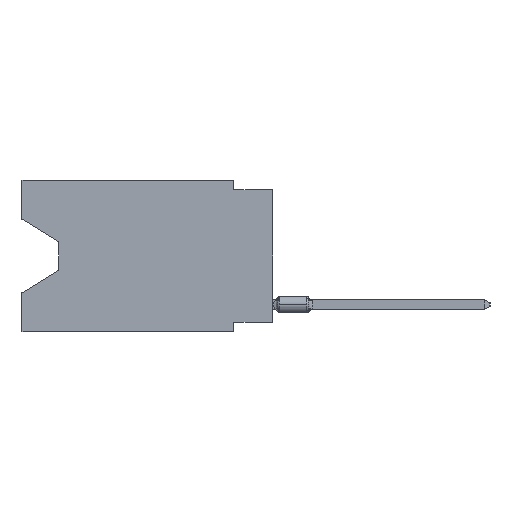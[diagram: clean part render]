
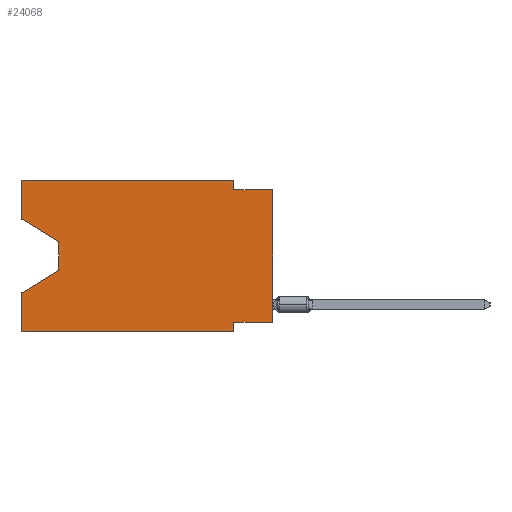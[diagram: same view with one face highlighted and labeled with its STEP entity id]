
A CAD part, left-side view. The second image highlights one B-rep face of the part: STEP entity #24068.
In plain terms, the highlighted planar face has unit normal (-1, 0, 0).
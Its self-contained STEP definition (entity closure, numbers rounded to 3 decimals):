
#17 = ORIENTED_EDGE ( 'NONE', *, *, #21297, .T. ) ;
#124 = VERTEX_POINT ( 'NONE', #58480 ) ;
#221 = VECTOR ( 'NONE', #21077, 1000. ) ;
#1026 = CARTESIAN_POINT ( 'NONE',  ( 0., 0., -0.635 ) ) ;
#1356 = LINE ( 'NONE', #67467, #20884 ) ;
#1847 = ORIENTED_EDGE ( 'NONE', *, *, #46155, .F. ) ;
#2629 = ORIENTED_EDGE ( 'NONE', *, *, #65726, .F. ) ;
#3691 = ORIENTED_EDGE ( 'NONE', *, *, #34728, .T. ) ;
#5023 = CARTESIAN_POINT ( 'NONE',  ( 0., 13.97, -5.893 ) ) ;
#10406 = CARTESIAN_POINT ( 'NONE',  ( 0., 13.97, -4.013 ) ) ;
#10746 = LINE ( 'NONE', #15737, #221 ) ;
#13681 = VERTEX_POINT ( 'NONE', #19581 ) ;
#15737 = CARTESIAN_POINT ( 'NONE',  ( 0., 16.383, -2.546 ) ) ;
#16040 = LINE ( 'NONE', #27062, #33808 ) ;
#17050 = EDGE_CURVE ( 'NONE', #27678, #64000, #19194, .T. ) ;
#17085 = CARTESIAN_POINT ( 'NONE',  ( 0., 0., -9.271 ) ) ;
#17692 = DIRECTION ( 'NONE',  ( 0., -1., 0. ) ) ;
#19194 = LINE ( 'NONE', #66882, #19429 ) ;
#19231 = DIRECTION ( 'NONE',  ( 0., 0., -1. ) ) ;
#19429 = VECTOR ( 'NONE', #57601, 1000. ) ;
#19581 = CARTESIAN_POINT ( 'NONE',  ( 0., 13.97, -4.013 ) ) ;
#20653 = DIRECTION ( 'NONE',  ( 0., 0., -1. ) ) ;
#20884 = VECTOR ( 'NONE', #17692, 1000. ) ;
#21077 = DIRECTION ( 'NONE',  ( 0., -0.855, -0.519 ) ) ;
#21142 = VECTOR ( 'NONE', #41375, 1000. ) ;
#21297 = EDGE_CURVE ( 'NONE', #68445, #124, #57919, .T. ) ;
#21388 = VERTEX_POINT ( 'NONE', #47588 ) ;
#21980 = EDGE_CURVE ( 'NONE', #68445, #21388, #50448, .T. ) ;
#21984 = VECTOR ( 'NONE', #36473, 1000. ) ;
#22849 = ORIENTED_EDGE ( 'NONE', *, *, #21980, .F. ) ;
#23095 = DIRECTION ( 'NONE',  ( 0., 0., 1. ) ) ;
#23615 = VERTEX_POINT ( 'NONE', #55124 ) ;
#23809 = EDGE_CURVE ( 'NONE', #13681, #24211, #70156, .T. ) ;
#24068 = ADVANCED_FACE ( 'NONE', ( #45902 ), #55889, .F. ) ;
#24211 = VERTEX_POINT ( 'NONE', #34907 ) ;
#25310 = DIRECTION ( 'NONE',  ( 0., 0.855, -0.519 ) ) ;
#25467 = EDGE_CURVE ( 'NONE', #29958, #57951, #69388, .T. ) ;
#25498 = VECTOR ( 'NONE', #25310, 1000. ) ;
#25687 = LINE ( 'NONE', #63403, #52208 ) ;
#27062 = CARTESIAN_POINT ( 'NONE',  ( 0., 2.54, -9.906 ) ) ;
#27487 = EDGE_LOOP ( 'NONE', ( #3691, #44027, #43756, #22849, #17, #68698, #41922, #69573, #2629, #48089, #1847, #38652 ) ) ;
#27678 = VERTEX_POINT ( 'NONE', #36654 ) ;
#27753 = VECTOR ( 'NONE', #23095, 1000. ) ;
#29958 = VERTEX_POINT ( 'NONE', #58519 ) ;
#30623 = EDGE_CURVE ( 'NONE', #63298, #23615, #44476, .T. ) ;
#32055 = LINE ( 'NONE', #5023, #25498 ) ;
#32377 = CARTESIAN_POINT ( 'NONE',  ( 0., 16.383, 0. ) ) ;
#33710 = CARTESIAN_POINT ( 'NONE',  ( 0., 16.383, -9.906 ) ) ;
#33808 = VECTOR ( 'NONE', #59084, 1000. ) ;
#34728 = EDGE_CURVE ( 'NONE', #27678, #13681, #10746, .T. ) ;
#34907 = CARTESIAN_POINT ( 'NONE',  ( 0., 13.97, -5.893 ) ) ;
#36473 = DIRECTION ( 'NONE',  ( 0., 0., 1. ) ) ;
#36654 = CARTESIAN_POINT ( 'NONE',  ( 0., 16.383, -2.546 ) ) ;
#36928 = CARTESIAN_POINT ( 'NONE',  ( 0., 16.383, -9.906 ) ) ;
#37163 = LINE ( 'NONE', #65257, #21984 ) ;
#37891 = VECTOR ( 'NONE', #68950, 1000. ) ;
#38652 = ORIENTED_EDGE ( 'NONE', *, *, #17050, .F. ) ;
#38673 = CARTESIAN_POINT ( 'NONE',  ( 0., 0., -9.271 ) ) ;
#41375 = DIRECTION ( 'NONE',  ( 0., 0., -1. ) ) ;
#41922 = ORIENTED_EDGE ( 'NONE', *, *, #30623, .F. ) ;
#43756 = ORIENTED_EDGE ( 'NONE', *, *, #66244, .T. ) ;
#44027 = ORIENTED_EDGE ( 'NONE', *, *, #23809, .T. ) ;
#44476 = LINE ( 'NONE', #17085, #60028 ) ;
#45902 = FACE_OUTER_BOUND ( 'NONE', #27487, .T. ) ;
#46155 = EDGE_CURVE ( 'NONE', #64000, #29958, #25687, .T. ) ;
#46250 = DIRECTION ( 'NONE',  ( 1., 0., 0. ) ) ;
#47370 = DIRECTION ( 'NONE',  ( 0., -1., 0. ) ) ;
#47588 = CARTESIAN_POINT ( 'NONE',  ( 0., 16.383, -7.36 ) ) ;
#47671 = CARTESIAN_POINT ( 'NONE',  ( 0., 2.54, 0. ) ) ;
#48089 = ORIENTED_EDGE ( 'NONE', *, *, #25467, .F. ) ;
#49818 = CARTESIAN_POINT ( 'NONE',  ( 0., 2.54, -0.635 ) ) ;
#50448 = LINE ( 'NONE', #55802, #27753 ) ;
#52208 = VECTOR ( 'NONE', #47370, 1000. ) ;
#53442 = EDGE_CURVE ( 'NONE', #23615, #124, #16040, .T. ) ;
#55124 = CARTESIAN_POINT ( 'NONE',  ( 0., 2.54, -9.271 ) ) ;
#55802 = CARTESIAN_POINT ( 'NONE',  ( 0., 16.383, 0. ) ) ;
#55889 = PLANE ( 'NONE',  #67745 ) ;
#57601 = DIRECTION ( 'NONE',  ( 0., 0., 1. ) ) ;
#57919 = LINE ( 'NONE', #36928, #37891 ) ;
#57951 = VERTEX_POINT ( 'NONE', #49818 ) ;
#58480 = CARTESIAN_POINT ( 'NONE',  ( 0., 2.54, -9.906 ) ) ;
#58519 = CARTESIAN_POINT ( 'NONE',  ( 0., 2.54, 0. ) ) ;
#59084 = DIRECTION ( 'NONE',  ( 0., 0., -1. ) ) ;
#60028 = VECTOR ( 'NONE', #65118, 1000. ) ;
#63006 = EDGE_CURVE ( 'NONE', #63298, #66802, #37163, .T. ) ;
#63298 = VERTEX_POINT ( 'NONE', #38673 ) ;
#63403 = CARTESIAN_POINT ( 'NONE',  ( 0., 16.383, 0. ) ) ;
#64000 = VERTEX_POINT ( 'NONE', #32377 ) ;
#64204 = VECTOR ( 'NONE', #20653, 1000. ) ;
#65118 = DIRECTION ( 'NONE',  ( 0., 1., 0. ) ) ;
#65257 = CARTESIAN_POINT ( 'NONE',  ( 0., 0., 0. ) ) ;
#65726 = EDGE_CURVE ( 'NONE', #57951, #66802, #1356, .T. ) ;
#66244 = EDGE_CURVE ( 'NONE', #24211, #21388, #32055, .T. ) ;
#66802 = VERTEX_POINT ( 'NONE', #1026 ) ;
#66882 = CARTESIAN_POINT ( 'NONE',  ( 0., 16.383, 0. ) ) ;
#67467 = CARTESIAN_POINT ( 'NONE',  ( 0., 0., -0.635 ) ) ;
#67601 = CARTESIAN_POINT ( 'NONE',  ( 0., 16.383, 0. ) ) ;
#67745 = AXIS2_PLACEMENT_3D ( 'NONE', #67601, #46250, #19231 ) ;
#68445 = VERTEX_POINT ( 'NONE', #33710 ) ;
#68698 = ORIENTED_EDGE ( 'NONE', *, *, #53442, .F. ) ;
#68950 = DIRECTION ( 'NONE',  ( 0., -1., 0. ) ) ;
#69388 = LINE ( 'NONE', #47671, #64204 ) ;
#69573 = ORIENTED_EDGE ( 'NONE', *, *, #63006, .T. ) ;
#70156 = LINE ( 'NONE', #10406, #21142 ) ;
